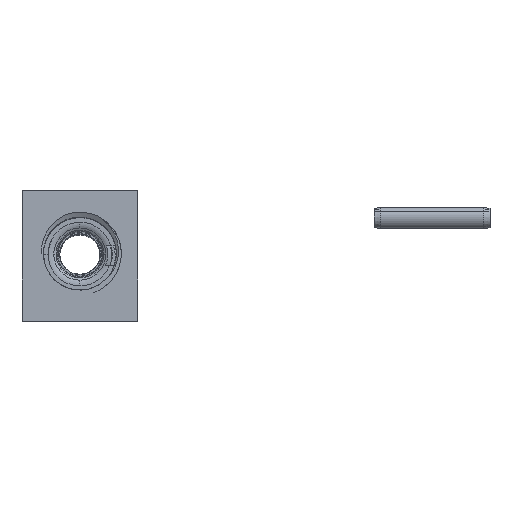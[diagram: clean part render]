
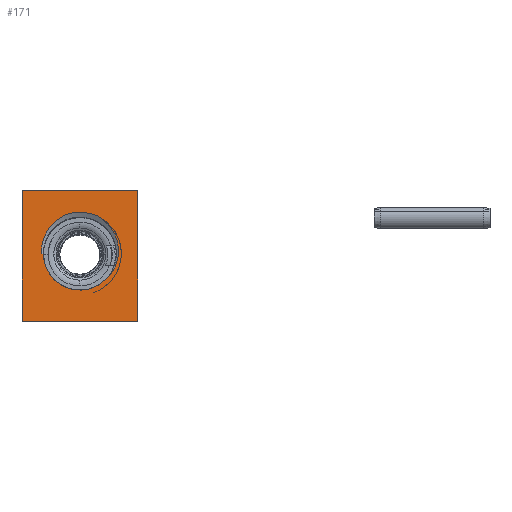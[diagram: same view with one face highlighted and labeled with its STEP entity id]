
A CAD part, top view. The second image highlights one B-rep face of the part: STEP entity #171.
In plain terms, the highlighted planar face has unit normal (0, 0, 1).
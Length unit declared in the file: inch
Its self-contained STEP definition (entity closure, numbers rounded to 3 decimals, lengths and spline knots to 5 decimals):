
#54 = CARTESIAN_POINT ( 'NONE',  ( 0., 0., 1.47 ) ) ;
#171 = ADVANCED_FACE ( 'NONE', ( #8536, #13635 ), #22293, .T. ) ;
#485 = CARTESIAN_POINT ( 'NONE',  ( 0.82888, -0.5635, 1.47 ) ) ;
#627 = CARTESIAN_POINT ( 'NONE',  ( 0.8345, -0.646, 1.47 ) ) ;
#746 = CARTESIAN_POINT ( 'NONE',  ( 0.24164, -0.41167, 1.47 ) ) ;
#765 = CARTESIAN_POINT ( 'NONE',  ( 0.79283, -0.45965, 1.47 ) ) ;
#913 = CARTESIAN_POINT ( 'NONE',  ( 0.83513, -0.61859, 1.47 ) ) ;
#1840 = LINE ( 'NONE', #54, #3879 ) ;
#1926 = ORIENTED_EDGE ( 'NONE', *, *, #7342, .T. ) ;
#2139 = CARTESIAN_POINT ( 'NONE',  ( 0., -0.6454, 1.47 ) ) ;
#2451 = AXIS2_PLACEMENT_3D ( 'NONE', #18659, #20611, #13886 ) ;
#2979 = CARTESIAN_POINT ( 'NONE',  ( 0.38401, -0.30716, 1.47 ) ) ;
#2999 = CARTESIAN_POINT ( 'NONE',  ( 0.80536, -0.48477, 1.47 ) ) ;
#3266 = CARTESIAN_POINT ( 'NONE',  ( 0.21256, -0.45688, 1.47 ) ) ;
#3693 = CARTESIAN_POINT ( 'NONE',  ( 0.65796, -0.3246, 1.47 ) ) ;
#3879 = VECTOR ( 'NONE', #22461, 39.37008 ) ;
#4264 = DIRECTION ( 'NONE',  ( 0., 1., 0. ) ) ;
#4373 = LINE ( 'NONE', #2139, #23361 ) ;
#4628 = EDGE_CURVE ( 'NONE', #20763, #5393, #4373, .T. ) ;
#4838 = CARTESIAN_POINT ( 'NONE',  ( 0., -1.23, 1.47 ) ) ;
#4991 = CARTESIAN_POINT ( 'NONE',  ( 0., -0.1, 1.47 ) ) ;
#5393 = VERTEX_POINT ( 'NONE', #10117 ) ;
#5526 = CARTESIAN_POINT ( 'NONE',  ( 0.80875, -0.75296, 1.47 ) ) ;
#5548 = EDGE_CURVE ( 'NONE', #20076, #5754, #24581, .T. ) ;
#5754 = VERTEX_POINT ( 'NONE', #25613 ) ;
#6243 = CARTESIAN_POINT ( 'NONE',  ( 0.47583, -0.28556, 1.47 ) ) ;
#6280 = ORIENTED_EDGE ( 'NONE', *, *, #25873, .T. ) ;
#6409 = B_SPLINE_CURVE_WITH_KNOTS ( 'NONE', 3,
 ( #23463, #11825, #11963, #26009, #16607, #20940, #21083, #765, #2999, #28245, #18712, #485, #27811, #913, #627, #18992, #28097, #9728, #5526, #16749, #19278, #25862, #23607, #12255, #14643 ),
 .UNSPECIFIED., .F., .F.,
 ( 4, 2, 2, 2, 2, 2, 2, 2, 2, 1, 2, 2, 4 ),
 ( 0., 0.0021, 0.00314, 0.00419, 0.00629, 0.00733, 0.00838, 0.01048, 0.01152, 0.01257, 0.01362, 0.01467, 0.01676 ),
 .UNSPECIFIED. ) ;
#7342 = EDGE_CURVE ( 'NONE', #19921, #20076, #13544, .T. ) ;
#7459 = CARTESIAN_POINT ( 'NONE',  ( 0.18402, -0.522, 1.47 ) ) ;
#8039 = CARTESIAN_POINT ( 'NONE',  ( 0.18985, -0.5052, 1.47 ) ) ;
#8156 = EDGE_CURVE ( 'NONE', #21529, #23437, #6409, .T. ) ;
#8536 = FACE_OUTER_BOUND ( 'NONE', #11092, .T. ) ;
#8561 = VERTEX_POINT ( 'NONE', #21470 ) ;
#8744 = B_SPLINE_CURVE_WITH_KNOTS ( 'NONE', 3,
 ( #10722, #19689, #6243, #11030, #28959, #17619 ),
 .UNSPECIFIED., .F., .F.,
 ( 4, 2, 4 ),
 ( 0., 0.00358, 0.00716 ),
 .UNSPECIFIED. ) ;
#9728 = CARTESIAN_POINT ( 'NONE',  ( 0.81791, -0.72707, 1.47 ) ) ;
#9850 = CARTESIAN_POINT ( 'NONE',  ( 0.32032, -0.33912, 1.47 ) ) ;
#9862 = CARTESIAN_POINT ( 'NONE',  ( 1., -1.23, 1.47 ) ) ;
#9865 = VECTOR ( 'NONE', #24313, 39.37008 ) ;
#10117 = CARTESIAN_POINT ( 'NONE',  ( 0.18504, -0.6454, 1.47 ) ) ;
#10138 = CARTESIAN_POINT ( 'NONE',  ( 0.17499, -0.55673, 1.47 ) ) ;
#10722 = CARTESIAN_POINT ( 'NONE',  ( 0.38401, -0.30716, 1.47 ) ) ;
#10916 = ORIENTED_EDGE ( 'NONE', *, *, #22595, .T. ) ;
#11030 = CARTESIAN_POINT ( 'NONE',  ( 0.56963, -0.29153, 1.47 ) ) ;
#11033 = EDGE_LOOP ( 'NONE', ( #10916, #16834, #25588, #16007, #6280 ) ) ;
#11092 = EDGE_LOOP ( 'NONE', ( #19014, #22528, #1926, #13118 ) ) ;
#11237 = DIRECTION ( 'NONE',  ( 0., 0., 1. ) ) ;
#11545 = EDGE_CURVE ( 'NONE', #5393, #23437, #29178, .T. ) ;
#11825 = CARTESIAN_POINT ( 'NONE',  ( 0.6821, -0.33837, 1.47 ) ) ;
#11963 = CARTESIAN_POINT ( 'NONE',  ( 0.70422, -0.35471, 1.47 ) ) ;
#12119 = CARTESIAN_POINT ( 'NONE',  ( 0.70795, -0.88195, 1.47 ) ) ;
#12255 = CARTESIAN_POINT ( 'NONE',  ( 0.73009, -0.86507, 1.47 ) ) ;
#12428 = VECTOR ( 'NONE', #4264, 39.37008 ) ;
#12650 = CARTESIAN_POINT ( 'NONE',  ( 0., -1.23, 1.47 ) ) ;
#12665 = CARTESIAN_POINT ( 'NONE',  ( 0., -0.1, 1.47 ) ) ;
#13118 = ORIENTED_EDGE ( 'NONE', *, *, #5548, .T. ) ;
#13544 = LINE ( 'NONE', #4838, #26307 ) ;
#13635 = FACE_BOUND ( 'NONE', #11033, .T. ) ;
#13886 = DIRECTION ( 'NONE',  ( 1., 0., 0. ) ) ;
#14106 = DIRECTION ( 'NONE',  ( 1., 0., 0. ) ) ;
#14475 = CARTESIAN_POINT ( 'NONE',  ( 0.35076, -0.32079, 1.47 ) ) ;
#14643 = CARTESIAN_POINT ( 'NONE',  ( 0.70795, -0.88195, 1.47 ) ) ;
#15878 = DIRECTION ( 'NONE',  ( 1., 0., 0. ) ) ;
#16007 = ORIENTED_EDGE ( 'NONE', *, *, #4628, .F. ) ;
#16607 = CARTESIAN_POINT ( 'NONE',  ( 0.74406, -0.39312, 1.47 ) ) ;
#16749 = CARTESIAN_POINT ( 'NONE',  ( 0.79643, -0.7775, 1.47 ) ) ;
#16834 = ORIENTED_EDGE ( 'NONE', *, *, #8156, .T. ) ;
#17260 = B_SPLINE_CURVE_WITH_KNOTS ( 'NONE', 3,
 ( #21648, #21500, #21352, #19399, #10138, #7459, #8039, #21067, #3266, #746, #23445, #9850, #14475, #2979 ),
 .UNSPECIFIED., .F., .F.,
 ( 4, 2, 2, 2, 2, 2, 4 ),
 ( 0., 0.00135, 0.00271, 0.00406, 0.00541, 0.00812, 0.01082 ),
 .UNSPECIFIED. ) ;
#17619 = CARTESIAN_POINT ( 'NONE',  ( 0.65796, -0.3246, 1.47 ) ) ;
#18659 = CARTESIAN_POINT ( 'NONE',  ( 0.5, -0.6454, 1.47 ) ) ;
#18712 = CARTESIAN_POINT ( 'NONE',  ( 0.8229, -0.53671, 1.47 ) ) ;
#18992 = CARTESIAN_POINT ( 'NONE',  ( 0.82838, -0.68683, 1.47 ) ) ;
#19014 = ORIENTED_EDGE ( 'NONE', *, *, #22784, .F. ) ;
#19278 = CARTESIAN_POINT ( 'NONE',  ( 0.78248, -0.80135, 1.47 ) ) ;
#19399 = CARTESIAN_POINT ( 'NONE',  ( 0.1719, -0.57432, 1.47 ) ) ;
#19689 = CARTESIAN_POINT ( 'NONE',  ( 0.42846, -0.29191, 1.47 ) ) ;
#19921 = VERTEX_POINT ( 'NONE', #12650 ) ;
#19987 = LINE ( 'NONE', #12665, #9865 ) ;
#20076 = VERTEX_POINT ( 'NONE', #9862 ) ;
#20611 = DIRECTION ( 'NONE',  ( 0., 0., 1. ) ) ;
#20730 = AXIS2_PLACEMENT_3D ( 'NONE', #22443, #11237, #15878 ) ;
#20763 = VERTEX_POINT ( 'NONE', #24884 ) ;
#20940 = CARTESIAN_POINT ( 'NONE',  ( 0.76185, -0.41422, 1.47 ) ) ;
#21067 = CARTESIAN_POINT ( 'NONE',  ( 0.2041, -0.47267, 1.47 ) ) ;
#21083 = CARTESIAN_POINT ( 'NONE',  ( 0.77009, -0.42523, 1.47 ) ) ;
#21352 = CARTESIAN_POINT ( 'NONE',  ( 0.16852, -0.60967, 1.47 ) ) ;
#21470 = CARTESIAN_POINT ( 'NONE',  ( 0.38401, -0.30716, 1.47 ) ) ;
#21500 = CARTESIAN_POINT ( 'NONE',  ( 0.16822, -0.62747, 1.47 ) ) ;
#21529 = VERTEX_POINT ( 'NONE', #3693 ) ;
#21648 = CARTESIAN_POINT ( 'NONE',  ( 0.16936, -0.6454, 1.47 ) ) ;
#22293 = PLANE ( 'NONE',  #20730 ) ;
#22443 = CARTESIAN_POINT ( 'NONE',  ( 0., 0., 1.47 ) ) ;
#22461 = DIRECTION ( 'NONE',  ( 0., -1., 0. ) ) ;
#22528 = ORIENTED_EDGE ( 'NONE', *, *, #28771, .T. ) ;
#22595 = EDGE_CURVE ( 'NONE', #8561, #21529, #8744, .T. ) ;
#22784 = EDGE_CURVE ( 'NONE', #24440, #5754, #19987, .T. ) ;
#23361 = VECTOR ( 'NONE', #29483, 39.37008 ) ;
#23437 = VERTEX_POINT ( 'NONE', #12119 ) ;
#23445 = CARTESIAN_POINT ( 'NONE',  ( 0.26512, -0.3851, 1.47 ) ) ;
#23463 = CARTESIAN_POINT ( 'NONE',  ( 0.65796, -0.3246, 1.47 ) ) ;
#23607 = CARTESIAN_POINT ( 'NONE',  ( 0.74947, -0.84564, 1.47 ) ) ;
#24313 = DIRECTION ( 'NONE',  ( 1., 0., 0. ) ) ;
#24440 = VERTEX_POINT ( 'NONE', #4991 ) ;
#24581 = LINE ( 'NONE', #26983, #12428 ) ;
#24884 = CARTESIAN_POINT ( 'NONE',  ( 0.16936, -0.6454, 1.47 ) ) ;
#25588 = ORIENTED_EDGE ( 'NONE', *, *, #11545, .F. ) ;
#25613 = CARTESIAN_POINT ( 'NONE',  ( 1., -0.1, 1.47 ) ) ;
#25862 = CARTESIAN_POINT ( 'NONE',  ( 0.77467, -0.81294, 1.47 ) ) ;
#25873 = EDGE_CURVE ( 'NONE', #20763, #8561, #17260, .T. ) ;
#26009 = CARTESIAN_POINT ( 'NONE',  ( 0.73445, -0.383, 1.47 ) ) ;
#26307 = VECTOR ( 'NONE', #14106, 39.37008 ) ;
#26983 = CARTESIAN_POINT ( 'NONE',  ( 1., 0., 1.47 ) ) ;
#27811 = CARTESIAN_POINT ( 'NONE',  ( 0.83108, -0.5772, 1.47 ) ) ;
#28097 = CARTESIAN_POINT ( 'NONE',  ( 0.82544, -0.70048, 1.47 ) ) ;
#28245 = CARTESIAN_POINT ( 'NONE',  ( 0.81911, -0.52355, 1.47 ) ) ;
#28771 = EDGE_CURVE ( 'NONE', #24440, #19921, #1840, .T. ) ;
#28959 = CARTESIAN_POINT ( 'NONE',  ( 0.61579, -0.30384, 1.47 ) ) ;
#29178 = CIRCLE ( 'NONE', #2451, 0.31496 ) ;
#29483 = DIRECTION ( 'NONE',  ( 1., 0., 0. ) ) ;
